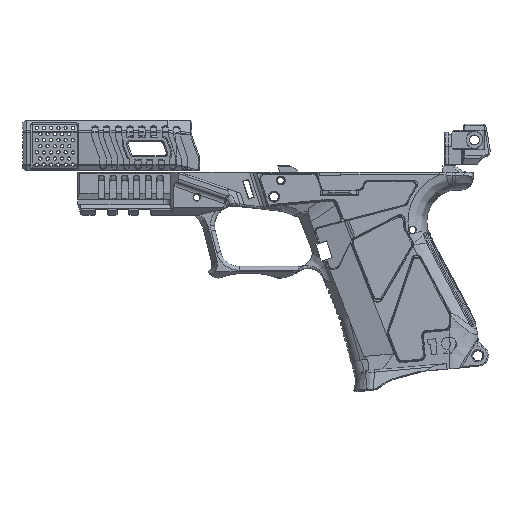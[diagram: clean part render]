
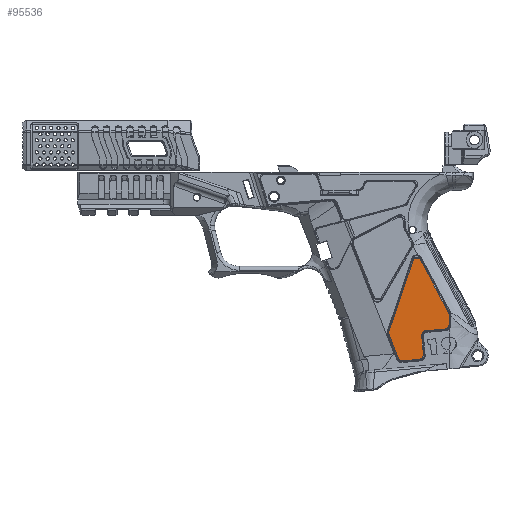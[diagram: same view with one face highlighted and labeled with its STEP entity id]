
A CAD part, top view. The second image highlights one B-rep face of the part: STEP entity #95536.
In plain terms, the highlighted face is planar.
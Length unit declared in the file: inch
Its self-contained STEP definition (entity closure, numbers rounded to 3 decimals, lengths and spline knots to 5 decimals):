
#145 = VERTEX_POINT ( 'NONE', #52652 ) ;
#418 = LINE ( 'NONE', #111984, #1529 ) ;
#980 = DIRECTION ( 'NONE',  ( 0., 0., -1. ) ) ;
#1054 = ORIENTED_EDGE ( 'NONE', *, *, #28028, .T. ) ;
#1464 = VECTOR ( 'NONE', #35625, 39.37008 ) ;
#1529 = VECTOR ( 'NONE', #9859, 39.37008 ) ;
#1912 = EDGE_CURVE ( 'NONE', #64904, #89998, #35560, .T. ) ;
#3159 = LINE ( 'NONE', #44423, #1464 ) ;
#5337 = AXIS2_PLACEMENT_3D ( 'NONE', #103382, #39835, #29030 ) ;
#8314 = ORIENTED_EDGE ( 'NONE', *, *, #109123, .F. ) ;
#8698 = EDGE_CURVE ( 'NONE', #89145, #131297, #111231, .T. ) ;
#9859 = DIRECTION ( 'NONE',  ( 0.089, 0.996, 0. ) ) ;
#9998 = AXIS2_PLACEMENT_3D ( 'NONE', #104649, #64090, #31661 ) ;
#11250 = VERTEX_POINT ( 'NONE', #16328 ) ;
#12410 = ORIENTED_EDGE ( 'NONE', *, *, #37542, .T. ) ;
#14173 = VECTOR ( 'NONE', #98594, 39.37008 ) ;
#14545 = AXIS2_PLACEMENT_3D ( 'NONE', #15808, #109091, #55725 ) ;
#15734 = DIRECTION ( 'NONE',  ( 0., 0., -1. ) ) ;
#15808 = CARTESIAN_POINT ( 'NONE',  ( 0.19818, -2.79663, -0.58693 ) ) ;
#16222 = CIRCLE ( 'NONE', #48655, 0.08 ) ;
#16328 = CARTESIAN_POINT ( 'NONE',  ( 0.11818, -2.79663, -0.58693 ) ) ;
#17469 = LINE ( 'NONE', #37710, #14173 ) ;
#18904 = CIRCLE ( 'NONE', #14545, 0.08 ) ;
#20476 = ORIENTED_EDGE ( 'NONE', *, *, #1912, .T. ) ;
#23819 = VERTEX_POINT ( 'NONE', #74986 ) ;
#24668 = DIRECTION ( 'NONE',  ( -0.996, 0.089, 0. ) ) ;
#28028 = EDGE_CURVE ( 'NONE', #145, #28510, #98522, .T. ) ;
#28510 = VERTEX_POINT ( 'NONE', #108067 ) ;
#28615 = VECTOR ( 'NONE', #127679, 39.37008 ) ;
#29030 = DIRECTION ( 'NONE',  ( -1., 0., 0. ) ) ;
#29328 = DIRECTION ( 'NONE',  ( 0., 0., -1. ) ) ;
#30210 = EDGE_CURVE ( 'NONE', #76192, #11250, #18904, .T. ) ;
#31552 = AXIS2_PLACEMENT_3D ( 'NONE', #73175, #31913, #92802 ) ;
#31661 = DIRECTION ( 'NONE',  ( -1., 0., 0. ) ) ;
#31913 = DIRECTION ( 'NONE',  ( 0., 0., -1. ) ) ;
#35006 = LINE ( 'NONE', #118857, #28615 ) ;
#35560 = CIRCLE ( 'NONE', #5337, 0.08 ) ;
#35625 = DIRECTION ( 'NONE',  ( -0.996, 0.089, 0. ) ) ;
#36818 = ORIENTED_EDGE ( 'NONE', *, *, #121304, .T. ) ;
#37542 = EDGE_CURVE ( 'NONE', #23819, #101652, #16222, .T. ) ;
#37710 = CARTESIAN_POINT ( 'NONE',  ( 0.11818, -2.86981, -0.58693 ) ) ;
#39464 = CARTESIAN_POINT ( 'NONE',  ( 0.69412, -1.68279, -0.58693 ) ) ;
#39835 = DIRECTION ( 'NONE',  ( 0., 0., -1. ) ) ;
#40100 = EDGE_CURVE ( 'NONE', #131297, #23819, #3159, .T. ) ;
#41659 = ORIENTED_EDGE ( 'NONE', *, *, #8698, .T. ) ;
#41712 = VECTOR ( 'NONE', #62617, 39.37008 ) ;
#42970 = CARTESIAN_POINT ( 'NONE',  ( 0.6162, -2.91426, -0.58693 ) ) ;
#43401 = VECTOR ( 'NONE', #54117, 39.37008 ) ;
#44423 = CARTESIAN_POINT ( 'NONE',  ( 1.01099, -3.45149, -0.58693 ) ) ;
#44615 = LINE ( 'NONE', #46620, #43401 ) ;
#44710 = CARTESIAN_POINT ( 'NONE',  ( 0.9585, -3.36649, -0.58693 ) ) ;
#46620 = CARTESIAN_POINT ( 'NONE',  ( 2.16018, -0.53411, -0.58693 ) ) ;
#47492 = ORIENTED_EDGE ( 'NONE', *, *, #63915, .T. ) ;
#48655 = AXIS2_PLACEMENT_3D ( 'NONE', #67267, #65936, #109165 ) ;
#48809 = EDGE_CURVE ( 'NONE', #28510, #54154, #35006, .T. ) ;
#51436 = CARTESIAN_POINT ( 'NONE',  ( 1.19653, -2.98048, -0.58693 ) ) ;
#51604 = CARTESIAN_POINT ( 'NONE',  ( 0.19107, -2.87632, -0.58693 ) ) ;
#52652 = CARTESIAN_POINT ( 'NONE',  ( 0.11818, -2.61552, -0.58693 ) ) ;
#53779 = LINE ( 'NONE', #42970, #77968 ) ;
#53801 = CARTESIAN_POINT ( 'NONE',  ( 1.1979, -2.92558, -0.58693 ) ) ;
#54117 = DIRECTION ( 'NONE',  ( -0.367, -0.93, 0. ) ) ;
#54154 = VERTEX_POINT ( 'NONE', #59598 ) ;
#55725 = DIRECTION ( 'NONE',  ( -1., 0., 0. ) ) ;
#56023 = VERTEX_POINT ( 'NONE', #104954 ) ;
#56971 = DIRECTION ( 'NONE',  ( -1., 0., 0. ) ) ;
#59598 = CARTESIAN_POINT ( 'NONE',  ( 0.62348, -1.64524, -0.58693 ) ) ;
#62617 = DIRECTION ( 'NONE',  ( -0.32, 0.948, 0. ) ) ;
#63778 = AXIS2_PLACEMENT_3D ( 'NONE', #44710, #980, #104428 ) ;
#63915 = EDGE_CURVE ( 'NONE', #56023, #76192, #53779, .T. ) ;
#64090 = DIRECTION ( 'NONE',  ( 0., 0., 1. ) ) ;
#64236 = EDGE_CURVE ( 'NONE', #89998, #89145, #44615, .T. ) ;
#64904 = VERTEX_POINT ( 'NONE', #53801 ) ;
#65936 = DIRECTION ( 'NONE',  ( 0., 0., -1. ) ) ;
#67267 = CARTESIAN_POINT ( 'NONE',  ( 0.65854, -3.33971, -0.58693 ) ) ;
#70562 = DIRECTION ( 'NONE',  ( -1., 0., 0. ) ) ;
#73175 = CARTESIAN_POINT ( 'NONE',  ( 0.19818, -2.61552, -0.58693 ) ) ;
#74099 = CARTESIAN_POINT ( 'NONE',  ( 1.20724, -2.95328, -0.58693 ) ) ;
#74518 = EDGE_CURVE ( 'NONE', #11250, #145, #17469, .T. ) ;
#74986 = CARTESIAN_POINT ( 'NONE',  ( 0.65143, -3.4194, -0.58693 ) ) ;
#75243 = ORIENTED_EDGE ( 'NONE', *, *, #97273, .T. ) ;
#76192 = VERTEX_POINT ( 'NONE', #51604 ) ;
#77968 = VECTOR ( 'NONE', #24668, 39.37008 ) ;
#82576 = ORIENTED_EDGE ( 'NONE', *, *, #48809, .T. ) ;
#83782 = ORIENTED_EDGE ( 'NONE', *, *, #40100, .T. ) ;
#85597 = CIRCLE ( 'NONE', #9998, 0.08 ) ;
#89145 = VERTEX_POINT ( 'NONE', #95632 ) ;
#89998 = VERTEX_POINT ( 'NONE', #51436 ) ;
#92771 = AXIS2_PLACEMENT_3D ( 'NONE', #39464, #29328, #70562 ) ;
#92802 = DIRECTION ( 'NONE',  ( -1., 0., 0. ) ) ;
#93069 = EDGE_LOOP ( 'NONE', ( #122455, #1054, #82576, #124660, #8314, #20476, #124751, #41659, #83782, #12410, #75243, #36818, #47492, #126739 ) ) ;
#95536 = ADVANCED_FACE ( 'NONE', ( #130675 ), #108358, .T. ) ;
#95632 = CARTESIAN_POINT ( 'NONE',  ( 1.03293, -3.39581, -0.58693 ) ) ;
#97273 = EDGE_CURVE ( 'NONE', #101652, #111648, #418, .T. ) ;
#98432 = AXIS2_PLACEMENT_3D ( 'NONE', #120524, #15734, #56971 ) ;
#98522 = CIRCLE ( 'NONE', #31552, 0.08 ) ;
#98594 = DIRECTION ( 'NONE',  ( 0., 1., 0. ) ) ;
#101652 = VERTEX_POINT ( 'NONE', #120843 ) ;
#103382 = CARTESIAN_POINT ( 'NONE',  ( 1.1221, -2.95116, -0.58693 ) ) ;
#104428 = DIRECTION ( 'NONE',  ( -1., 0., 0. ) ) ;
#104649 = CARTESIAN_POINT ( 'NONE',  ( 0.5294, -2.98683, -0.58693 ) ) ;
#104954 = CARTESIAN_POINT ( 'NONE',  ( 0.53652, -2.90715, -0.58693 ) ) ;
#105662 = CIRCLE ( 'NONE', #92771, 0.08 ) ;
#108067 = CARTESIAN_POINT ( 'NONE',  ( 0.12754, -2.57796, -0.58693 ) ) ;
#108358 = PLANE ( 'NONE',  #98432 ) ;
#109091 = DIRECTION ( 'NONE',  ( 0., 0., -1. ) ) ;
#109123 = EDGE_CURVE ( 'NONE', #64904, #128678, #126805, .T. ) ;
#109165 = DIRECTION ( 'NONE',  ( -1., 0., 0. ) ) ;
#111231 = CIRCLE ( 'NONE', #63778, 0.08 ) ;
#111648 = VERTEX_POINT ( 'NONE', #128880 ) ;
#111984 = CARTESIAN_POINT ( 'NONE',  ( 0.57174, -3.41228, -0.58693 ) ) ;
#113430 = CARTESIAN_POINT ( 'NONE',  ( 0.76992, -1.65722, -0.58693 ) ) ;
#118857 = CARTESIAN_POINT ( 'NONE',  ( 0.11818, -2.59557, -0.58693 ) ) ;
#120524 = CARTESIAN_POINT ( 'NONE',  ( 0.81474, -0.46842, -0.58693 ) ) ;
#120843 = CARTESIAN_POINT ( 'NONE',  ( 0.57886, -3.3326, -0.58693 ) ) ;
#121304 = EDGE_CURVE ( 'NONE', #111648, #56023, #85597, .T. ) ;
#122455 = ORIENTED_EDGE ( 'NONE', *, *, #74518, .T. ) ;
#124660 = ORIENTED_EDGE ( 'NONE', *, *, #130487, .T. ) ;
#124690 = CARTESIAN_POINT ( 'NONE',  ( 0.95138, -3.44617, -0.58693 ) ) ;
#124751 = ORIENTED_EDGE ( 'NONE', *, *, #64236, .T. ) ;
#126739 = ORIENTED_EDGE ( 'NONE', *, *, #30210, .T. ) ;
#126805 = LINE ( 'NONE', #74099, #41712 ) ;
#127679 = DIRECTION ( 'NONE',  ( 0.469, 0.883, 0. ) ) ;
#128678 = VERTEX_POINT ( 'NONE', #113430 ) ;
#128880 = CARTESIAN_POINT ( 'NONE',  ( 0.60909, -2.99395, -0.58693 ) ) ;
#130487 = EDGE_CURVE ( 'NONE', #54154, #128678, #105662, .T. ) ;
#130675 = FACE_OUTER_BOUND ( 'NONE', #93069, .T. ) ;
#131297 = VERTEX_POINT ( 'NONE', #124690 ) ;
